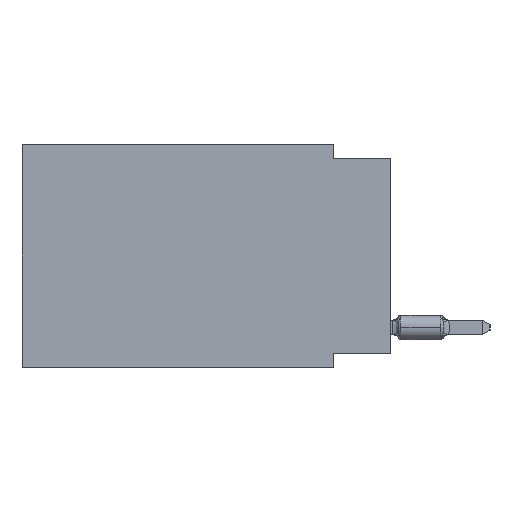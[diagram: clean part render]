
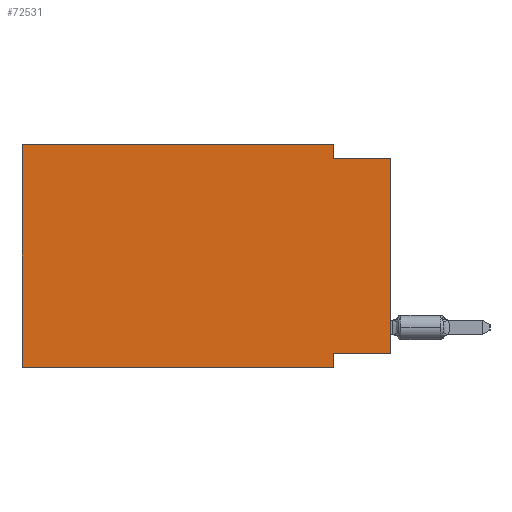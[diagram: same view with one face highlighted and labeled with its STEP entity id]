
A CAD part, left-side view. The second image highlights one B-rep face of the part: STEP entity #72531.
In plain terms, the highlighted planar face has unit normal (-1, 0, 0).
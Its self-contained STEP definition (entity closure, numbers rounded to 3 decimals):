
#895 = LINE ( 'NONE', #47190, #28992 ) ;
#3221 = EDGE_CURVE ( 'NONE', #5225, #62079, #895, .T. ) ;
#5225 = VERTEX_POINT ( 'NONE', #48623 ) ;
#6545 = EDGE_CURVE ( 'NONE', #28102, #8007, #20770, .T. ) ;
#6849 = VERTEX_POINT ( 'NONE', #33093 ) ;
#7087 = VERTEX_POINT ( 'NONE', #30417 ) ;
#8007 = VERTEX_POINT ( 'NONE', #71138 ) ;
#10218 = CARTESIAN_POINT ( 'NONE',  ( 0., 2.54, -9.271 ) ) ;
#10570 = DIRECTION ( 'NONE',  ( 0., -1., 0. ) ) ;
#10588 = CARTESIAN_POINT ( 'NONE',  ( 0., 2.54, -9.906 ) ) ;
#10839 = CARTESIAN_POINT ( 'NONE',  ( 0., 16.383, 0. ) ) ;
#11039 = ORIENTED_EDGE ( 'NONE', *, *, #18951, .T. ) ;
#11519 = VECTOR ( 'NONE', #29581, 1000. ) ;
#12107 = CARTESIAN_POINT ( 'NONE',  ( 0., 16.383, 0. ) ) ;
#12255 = EDGE_CURVE ( 'NONE', #7087, #28102, #34108, .T. ) ;
#12798 = DIRECTION ( 'NONE',  ( 0., 0., 1. ) ) ;
#15148 = DIRECTION ( 'NONE',  ( 0., 0., 1. ) ) ;
#16498 = AXIS2_PLACEMENT_3D ( 'NONE', #60384, #20118, #26142 ) ;
#18043 = EDGE_CURVE ( 'NONE', #34580, #6849, #24726, .T. ) ;
#18951 = EDGE_CURVE ( 'NONE', #7087, #38272, #29366, .T. ) ;
#20118 = DIRECTION ( 'NONE',  ( 1., 0., 0. ) ) ;
#20770 = LINE ( 'NONE', #10588, #23316 ) ;
#20866 = VECTOR ( 'NONE', #10570, 1000. ) ;
#22233 = CARTESIAN_POINT ( 'NONE',  ( 0., 16.383, -9.906 ) ) ;
#23316 = VECTOR ( 'NONE', #73806, 1000. ) ;
#24726 = LINE ( 'NONE', #64619, #51614 ) ;
#26142 = DIRECTION ( 'NONE',  ( 0., 0., -1. ) ) ;
#26911 = ORIENTED_EDGE ( 'NONE', *, *, #57691, .F. ) ;
#27252 = PLANE ( 'NONE',  #16498 ) ;
#27263 = EDGE_CURVE ( 'NONE', #62079, #34580, #47103, .T. ) ;
#28102 = VERTEX_POINT ( 'NONE', #10218 ) ;
#28823 = CARTESIAN_POINT ( 'NONE',  ( 0., 0., -9.271 ) ) ;
#28992 = VECTOR ( 'NONE', #15148, 1000. ) ;
#29366 = LINE ( 'NONE', #64708, #72095 ) ;
#29581 = DIRECTION ( 'NONE',  ( 0., 1., 0. ) ) ;
#30417 = CARTESIAN_POINT ( 'NONE',  ( 0., 0., -9.271 ) ) ;
#32152 = CARTESIAN_POINT ( 'NONE',  ( 0., 0., -0.635 ) ) ;
#33093 = CARTESIAN_POINT ( 'NONE',  ( 0., 2.54, -0.635 ) ) ;
#34108 = LINE ( 'NONE', #28823, #11519 ) ;
#34580 = VERTEX_POINT ( 'NONE', #63400 ) ;
#38272 = VERTEX_POINT ( 'NONE', #42198 ) ;
#39149 = VECTOR ( 'NONE', #50559, 1000. ) ;
#39278 = LINE ( 'NONE', #32152, #39149 ) ;
#41238 = ORIENTED_EDGE ( 'NONE', *, *, #67740, .T. ) ;
#41522 = ORIENTED_EDGE ( 'NONE', *, *, #18043, .F. ) ;
#42198 = CARTESIAN_POINT ( 'NONE',  ( 0., 0., -0.635 ) ) ;
#42583 = ORIENTED_EDGE ( 'NONE', *, *, #6545, .F. ) ;
#43307 = ORIENTED_EDGE ( 'NONE', *, *, #3221, .F. ) ;
#44084 = LINE ( 'NONE', #22233, #20866 ) ;
#44521 = ORIENTED_EDGE ( 'NONE', *, *, #27263, .F. ) ;
#47003 = ORIENTED_EDGE ( 'NONE', *, *, #12255, .F. ) ;
#47103 = LINE ( 'NONE', #12107, #57329 ) ;
#47190 = CARTESIAN_POINT ( 'NONE',  ( 0., 16.383, 0. ) ) ;
#48623 = CARTESIAN_POINT ( 'NONE',  ( 0., 16.383, -9.906 ) ) ;
#50559 = DIRECTION ( 'NONE',  ( 0., -1., 0. ) ) ;
#51614 = VECTOR ( 'NONE', #53312, 1000. ) ;
#51616 = EDGE_LOOP ( 'NONE', ( #11039, #26911, #41522, #44521, #43307, #41238, #42583, #47003 ) ) ;
#53312 = DIRECTION ( 'NONE',  ( 0., 0., -1. ) ) ;
#57329 = VECTOR ( 'NONE', #70061, 1000. ) ;
#57691 = EDGE_CURVE ( 'NONE', #6849, #38272, #39278, .T. ) ;
#60384 = CARTESIAN_POINT ( 'NONE',  ( 0., 16.383, 0. ) ) ;
#62079 = VERTEX_POINT ( 'NONE', #10839 ) ;
#63400 = CARTESIAN_POINT ( 'NONE',  ( 0., 2.54, 0. ) ) ;
#64619 = CARTESIAN_POINT ( 'NONE',  ( 0., 2.54, 0. ) ) ;
#64708 = CARTESIAN_POINT ( 'NONE',  ( 0., 0., 0. ) ) ;
#67740 = EDGE_CURVE ( 'NONE', #5225, #8007, #44084, .T. ) ;
#70061 = DIRECTION ( 'NONE',  ( 0., -1., 0. ) ) ;
#71138 = CARTESIAN_POINT ( 'NONE',  ( 0., 2.54, -9.906 ) ) ;
#71676 = FACE_OUTER_BOUND ( 'NONE', #51616, .T. ) ;
#72095 = VECTOR ( 'NONE', #12798, 1000. ) ;
#72531 = ADVANCED_FACE ( 'NONE', ( #71676 ), #27252, .F. ) ;
#73806 = DIRECTION ( 'NONE',  ( 0., 0., -1. ) ) ;
